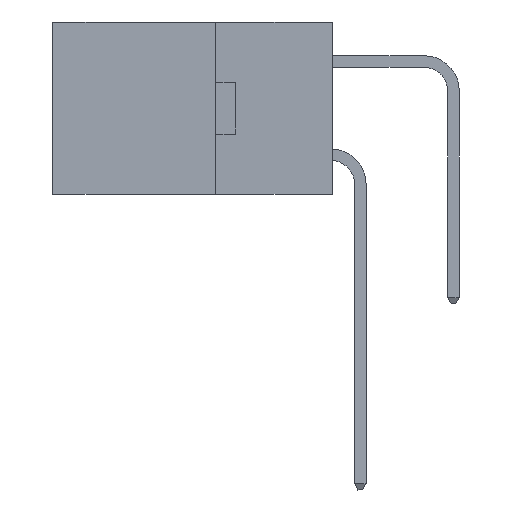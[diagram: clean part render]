
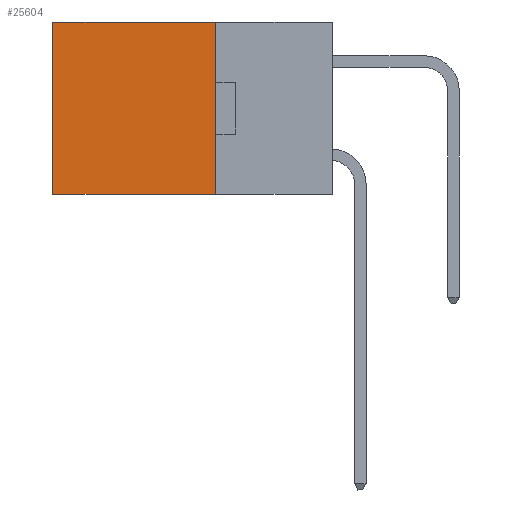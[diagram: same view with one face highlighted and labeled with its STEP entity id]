
A CAD part, left-side view. The second image highlights one B-rep face of the part: STEP entity #25604.
In plain terms, the highlighted planar face has unit normal (-1, 0, 0).
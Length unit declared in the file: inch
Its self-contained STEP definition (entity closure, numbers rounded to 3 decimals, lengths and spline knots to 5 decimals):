
#464 = VERTEX_POINT ( 'NONE', #5731 ) ;
#1237 = CARTESIAN_POINT ( 'NONE',  ( 0.2615, 0.25, 0. ) ) ;
#1923 = AXIS2_PLACEMENT_3D ( 'NONE', #5417, #28500, #14695 ) ;
#1941 = ORIENTED_EDGE ( 'NONE', *, *, #18081, .F. ) ;
#2118 = DIRECTION ( 'NONE',  ( 0., 0., -1. ) ) ;
#3614 = DIRECTION ( 'NONE',  ( 0., 1., 0. ) ) ;
#3851 = EDGE_LOOP ( 'NONE', ( #21284, #12006, #1941, #25062 ) ) ;
#4657 = CARTESIAN_POINT ( 'NONE',  ( 0.2615, 0.6, -0.37 ) ) ;
#5417 = CARTESIAN_POINT ( 'NONE',  ( 0.2615, 0.25, -0.37 ) ) ;
#5731 = CARTESIAN_POINT ( 'NONE',  ( 0.2615, 0.25, -0.37 ) ) ;
#6014 = CARTESIAN_POINT ( 'NONE',  ( 0.2615, 0.6, -0.37 ) ) ;
#6039 = DIRECTION ( 'NONE',  ( 0., 1., 0. ) ) ;
#6858 = CARTESIAN_POINT ( 'NONE',  ( 0.2615, 0.6, 0. ) ) ;
#7369 = LINE ( 'NONE', #29812, #19635 ) ;
#8377 = FACE_OUTER_BOUND ( 'NONE', #3851, .T. ) ;
#8594 = VERTEX_POINT ( 'NONE', #12510 ) ;
#10587 = CARTESIAN_POINT ( 'NONE',  ( 0.2615, 0.25, -0.37 ) ) ;
#10895 = LINE ( 'NONE', #6014, #23173 ) ;
#10914 = VERTEX_POINT ( 'NONE', #6858 ) ;
#12006 = ORIENTED_EDGE ( 'NONE', *, *, #24910, .F. ) ;
#12377 = PLANE ( 'NONE',  #1923 ) ;
#12510 = CARTESIAN_POINT ( 'NONE',  ( 0.2615, 0.25, 0. ) ) ;
#13035 = LINE ( 'NONE', #10587, #24596 ) ;
#14587 = VECTOR ( 'NONE', #3614, 39.37008 ) ;
#14695 = DIRECTION ( 'NONE',  ( 0., 0., -1. ) ) ;
#17795 = EDGE_CURVE ( 'NONE', #8594, #10914, #26870, .T. ) ;
#18081 = EDGE_CURVE ( 'NONE', #8594, #464, #7369, .T. ) ;
#19265 = EDGE_CURVE ( 'NONE', #10914, #27698, #10895, .T. ) ;
#19635 = VECTOR ( 'NONE', #2118, 39.37008 ) ;
#21284 = ORIENTED_EDGE ( 'NONE', *, *, #19265, .T. ) ;
#22192 = DIRECTION ( 'NONE',  ( 0., 0., -1. ) ) ;
#23173 = VECTOR ( 'NONE', #22192, 39.37008 ) ;
#24596 = VECTOR ( 'NONE', #6039, 39.37008 ) ;
#24910 = EDGE_CURVE ( 'NONE', #464, #27698, #13035, .T. ) ;
#25062 = ORIENTED_EDGE ( 'NONE', *, *, #17795, .T. ) ;
#25604 = ADVANCED_FACE ( 'NONE', ( #8377 ), #12377, .F. ) ;
#26870 = LINE ( 'NONE', #1237, #14587 ) ;
#27698 = VERTEX_POINT ( 'NONE', #4657 ) ;
#28500 = DIRECTION ( 'NONE',  ( 1., 0., 0. ) ) ;
#29812 = CARTESIAN_POINT ( 'NONE',  ( 0.2615, 0.25, -0.37 ) ) ;
